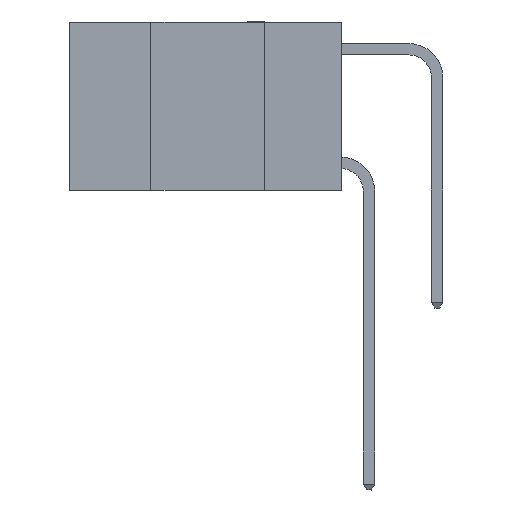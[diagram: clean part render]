
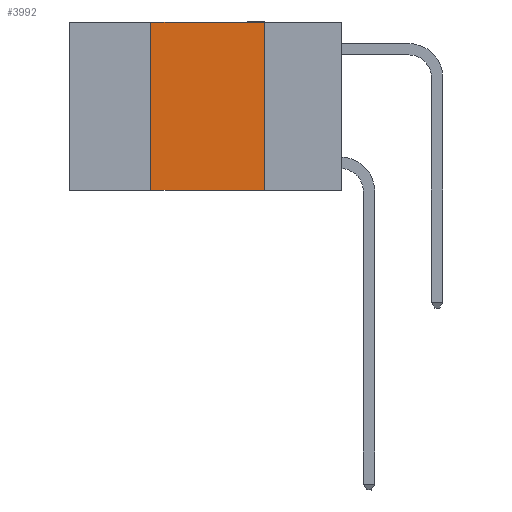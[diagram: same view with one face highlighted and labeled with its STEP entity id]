
A CAD part, left-side view. The second image highlights one B-rep face of the part: STEP entity #3992.
In plain terms, the highlighted planar face has unit normal (-1, 0, 0).
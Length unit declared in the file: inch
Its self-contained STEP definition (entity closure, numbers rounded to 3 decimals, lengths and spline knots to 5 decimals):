
#64 = CARTESIAN_POINT ( 'NONE',  ( 0., 0.6, -0.37 ) ) ;
#195 = EDGE_CURVE ( 'NONE', #12717, #1048, #8464, .T. ) ;
#513 = DIRECTION ( 'NONE',  ( 0., -1., 0. ) ) ;
#1048 = VERTEX_POINT ( 'NONE', #13359 ) ;
#1053 = CARTESIAN_POINT ( 'NONE',  ( 0., 0.17, 0. ) ) ;
#1880 = LINE ( 'NONE', #10892, #2203 ) ;
#1894 = FACE_OUTER_BOUND ( 'NONE', #9315, .T. ) ;
#2203 = VECTOR ( 'NONE', #7955, 39.37008 ) ;
#2242 = DIRECTION ( 'NONE',  ( 0., 0., -1. ) ) ;
#2732 = CARTESIAN_POINT ( 'NONE',  ( 0., 0.6, 0. ) ) ;
#3795 = DIRECTION ( 'NONE',  ( 1., 0., 0. ) ) ;
#3931 = CARTESIAN_POINT ( 'NONE',  ( 0., 0.42, 0. ) ) ;
#3992 = ADVANCED_FACE ( 'NONE', ( #1894 ), #9039, .F. ) ;
#4261 = EDGE_CURVE ( 'NONE', #7953, #5314, #1880, .T. ) ;
#4284 = VECTOR ( 'NONE', #2242, 39.37008 ) ;
#4520 = ORIENTED_EDGE ( 'NONE', *, *, #6226, .F. ) ;
#4715 = ORIENTED_EDGE ( 'NONE', *, *, #6826, .F. ) ;
#4841 = ORIENTED_EDGE ( 'NONE', *, *, #195, .T. ) ;
#5314 = VERTEX_POINT ( 'NONE', #8445 ) ;
#5409 = VECTOR ( 'NONE', #11113, 39.37008 ) ;
#5720 = LINE ( 'NONE', #3931, #5409 ) ;
#6226 = EDGE_CURVE ( 'NONE', #5314, #1048, #7479, .T. ) ;
#6826 = EDGE_CURVE ( 'NONE', #12717, #7953, #5720, .T. ) ;
#7479 = LINE ( 'NONE', #1053, #4284 ) ;
#7953 = VERTEX_POINT ( 'NONE', #12092 ) ;
#7955 = DIRECTION ( 'NONE',  ( 0., -1., 0. ) ) ;
#8288 = CARTESIAN_POINT ( 'NONE',  ( 0., 0.42, -0.37 ) ) ;
#8445 = CARTESIAN_POINT ( 'NONE',  ( 0., 0.17, 0. ) ) ;
#8464 = LINE ( 'NONE', #64, #11068 ) ;
#9039 = PLANE ( 'NONE',  #10153 ) ;
#9315 = EDGE_LOOP ( 'NONE', ( #4520, #9618, #4715, #4841 ) ) ;
#9618 = ORIENTED_EDGE ( 'NONE', *, *, #4261, .F. ) ;
#10153 = AXIS2_PLACEMENT_3D ( 'NONE', #2732, #3795, #10985 ) ;
#10892 = CARTESIAN_POINT ( 'NONE',  ( 0., 0.6, 0. ) ) ;
#10985 = DIRECTION ( 'NONE',  ( 0., 0., -1. ) ) ;
#11068 = VECTOR ( 'NONE', #513, 39.37008 ) ;
#11113 = DIRECTION ( 'NONE',  ( 0., 0., 1. ) ) ;
#12092 = CARTESIAN_POINT ( 'NONE',  ( 0., 0.42, 0. ) ) ;
#12717 = VERTEX_POINT ( 'NONE', #8288 ) ;
#13359 = CARTESIAN_POINT ( 'NONE',  ( 0., 0.17, -0.37 ) ) ;
